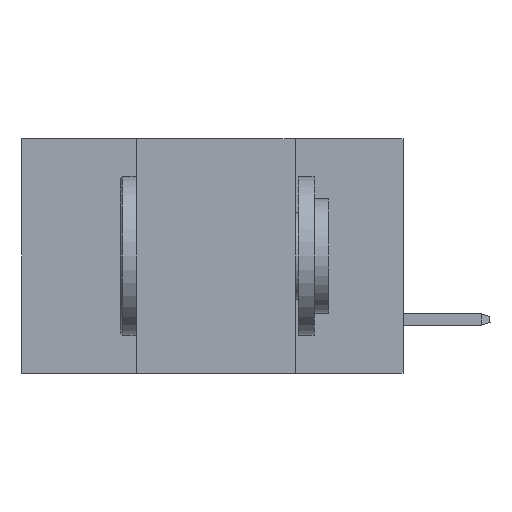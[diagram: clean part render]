
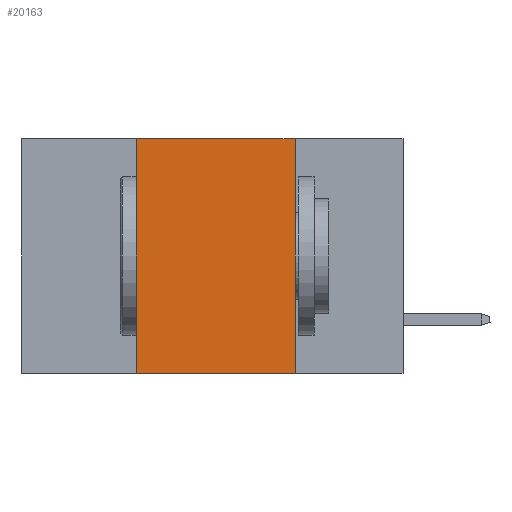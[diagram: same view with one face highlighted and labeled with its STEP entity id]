
A CAD part, left-side view. The second image highlights one B-rep face of the part: STEP entity #20163.
In plain terms, the highlighted planar face has unit normal (-1, 0, 0).
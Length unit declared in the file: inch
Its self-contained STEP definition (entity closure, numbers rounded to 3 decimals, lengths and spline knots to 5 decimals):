
#92 = LINE ( 'NONE', #9123, #1930 ) ;
#1930 = VECTOR ( 'NONE', #18074, 39.37008 ) ;
#2321 = VECTOR ( 'NONE', #10879, 39.37008 ) ;
#2870 = AXIS2_PLACEMENT_3D ( 'NONE', #11982, #19143, #10451 ) ;
#3468 = CARTESIAN_POINT ( 'NONE',  ( 0., 0.42, 0. ) ) ;
#4145 = ORIENTED_EDGE ( 'NONE', *, *, #5678, .F. ) ;
#4812 = LINE ( 'NONE', #12104, #10634 ) ;
#4987 = CARTESIAN_POINT ( 'NONE',  ( 0., 0.17, -0.37 ) ) ;
#5678 = EDGE_CURVE ( 'NONE', #9281, #11287, #92, .T. ) ;
#5954 = LINE ( 'NONE', #18641, #15202 ) ;
#6059 = ORIENTED_EDGE ( 'NONE', *, *, #6101, .F. ) ;
#6101 = EDGE_CURVE ( 'NONE', #21365, #20689, #12286, .T. ) ;
#6697 = EDGE_LOOP ( 'NONE', ( #4145, #10219, #6059, #20296 ) ) ;
#9107 = EDGE_CURVE ( 'NONE', #20689, #9281, #4812, .T. ) ;
#9123 = CARTESIAN_POINT ( 'NONE',  ( 0., 0.17, 0. ) ) ;
#9281 = VERTEX_POINT ( 'NONE', #13161 ) ;
#9516 = CARTESIAN_POINT ( 'NONE',  ( 0., 0.42, -0.37 ) ) ;
#10219 = ORIENTED_EDGE ( 'NONE', *, *, #9107, .F. ) ;
#10451 = DIRECTION ( 'NONE',  ( 0., 0., -1. ) ) ;
#10634 = VECTOR ( 'NONE', #19259, 39.37008 ) ;
#10879 = DIRECTION ( 'NONE',  ( 0., 0., 1. ) ) ;
#10936 = EDGE_CURVE ( 'NONE', #21365, #11287, #5954, .T. ) ;
#11287 = VERTEX_POINT ( 'NONE', #4987 ) ;
#11488 = DIRECTION ( 'NONE',  ( 0., -1., 0. ) ) ;
#11982 = CARTESIAN_POINT ( 'NONE',  ( 0., 0.6, 0. ) ) ;
#12104 = CARTESIAN_POINT ( 'NONE',  ( 0., 0.6, 0. ) ) ;
#12286 = LINE ( 'NONE', #19443, #2321 ) ;
#13161 = CARTESIAN_POINT ( 'NONE',  ( 0., 0.17, 0. ) ) ;
#15202 = VECTOR ( 'NONE', #11488, 39.37008 ) ;
#15502 = FACE_OUTER_BOUND ( 'NONE', #6697, .T. ) ;
#18074 = DIRECTION ( 'NONE',  ( 0., 0., -1. ) ) ;
#18641 = CARTESIAN_POINT ( 'NONE',  ( 0., 0.6, -0.37 ) ) ;
#19143 = DIRECTION ( 'NONE',  ( 1., 0., 0. ) ) ;
#19259 = DIRECTION ( 'NONE',  ( 0., -1., 0. ) ) ;
#19443 = CARTESIAN_POINT ( 'NONE',  ( 0., 0.42, 0. ) ) ;
#20163 = ADVANCED_FACE ( 'NONE', ( #15502 ), #20895, .F. ) ;
#20296 = ORIENTED_EDGE ( 'NONE', *, *, #10936, .T. ) ;
#20689 = VERTEX_POINT ( 'NONE', #3468 ) ;
#20895 = PLANE ( 'NONE',  #2870 ) ;
#21365 = VERTEX_POINT ( 'NONE', #9516 ) ;
